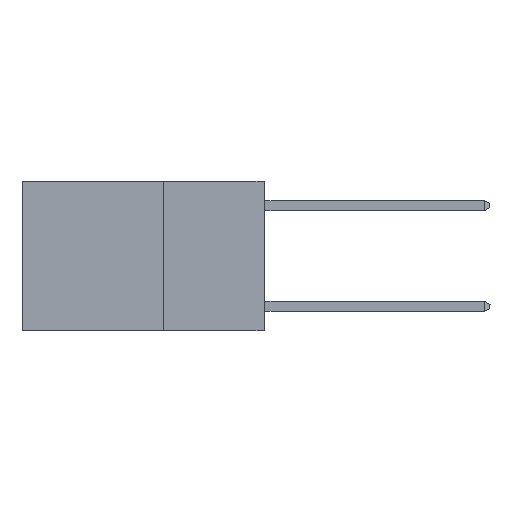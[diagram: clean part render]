
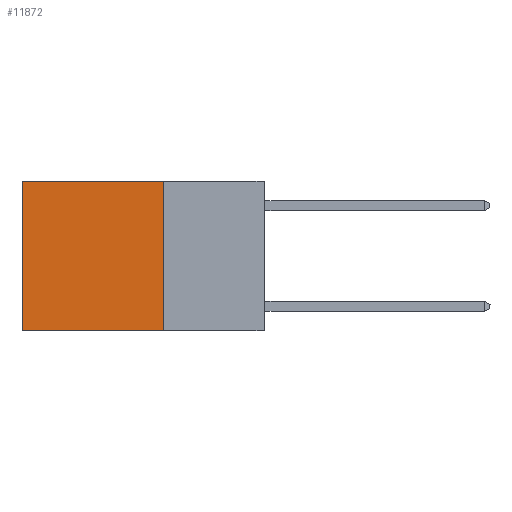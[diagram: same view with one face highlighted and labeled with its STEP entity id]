
A CAD part, left-side view. The second image highlights one B-rep face of the part: STEP entity #11872.
In plain terms, the highlighted planar face has unit normal (-1, 0, 0).
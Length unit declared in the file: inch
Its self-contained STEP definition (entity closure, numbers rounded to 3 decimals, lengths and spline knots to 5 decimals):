
#581 = LINE ( 'NONE', #2000, #25462 ) ;
#1449 = PLANE ( 'NONE',  #12450 ) ;
#1751 = DIRECTION ( 'NONE',  ( 0., 1., 0. ) ) ;
#1859 = LINE ( 'NONE', #28001, #8351 ) ;
#2000 = CARTESIAN_POINT ( 'NONE',  ( 0.2625, 0.6, 0. ) ) ;
#2267 = LINE ( 'NONE', #19824, #20061 ) ;
#4244 = EDGE_CURVE ( 'NONE', #11460, #20288, #2267, .T. ) ;
#4685 = VERTEX_POINT ( 'NONE', #14009 ) ;
#4867 = ORIENTED_EDGE ( 'NONE', *, *, #16510, .T. ) ;
#6562 = CARTESIAN_POINT ( 'NONE',  ( 0.2625, 0.25, 0. ) ) ;
#6848 = VECTOR ( 'NONE', #1751, 39.37008 ) ;
#7389 = FACE_OUTER_BOUND ( 'NONE', #16696, .T. ) ;
#8351 = VECTOR ( 'NONE', #20882, 39.37008 ) ;
#8789 = CARTESIAN_POINT ( 'NONE',  ( 0.2625, 0.25, 0. ) ) ;
#9320 = DIRECTION ( 'NONE',  ( 0., 0., -1. ) ) ;
#10225 = DIRECTION ( 'NONE',  ( 0., 1., 0. ) ) ;
#11220 = DIRECTION ( 'NONE',  ( 1., 0., 0. ) ) ;
#11307 = CARTESIAN_POINT ( 'NONE',  ( 0.2625, 0.6, -0.37 ) ) ;
#11460 = VERTEX_POINT ( 'NONE', #19365 ) ;
#11872 = ADVANCED_FACE ( 'NONE', ( #7389 ), #1449, .F. ) ;
#12450 = AXIS2_PLACEMENT_3D ( 'NONE', #8789, #11220, #27911 ) ;
#12528 = ORIENTED_EDGE ( 'NONE', *, *, #4244, .F. ) ;
#13255 = LINE ( 'NONE', #6562, #6848 ) ;
#14009 = CARTESIAN_POINT ( 'NONE',  ( 0.2625, 0.25, 0. ) ) ;
#14390 = EDGE_CURVE ( 'NONE', #4685, #11460, #1859, .T. ) ;
#14433 = EDGE_CURVE ( 'NONE', #4685, #24748, #13255, .T. ) ;
#16510 = EDGE_CURVE ( 'NONE', #24748, #20288, #581, .T. ) ;
#16696 = EDGE_LOOP ( 'NONE', ( #4867, #12528, #22081, #19444 ) ) ;
#19365 = CARTESIAN_POINT ( 'NONE',  ( 0.2625, 0.25, -0.37 ) ) ;
#19444 = ORIENTED_EDGE ( 'NONE', *, *, #14433, .T. ) ;
#19824 = CARTESIAN_POINT ( 'NONE',  ( 0.2625, 0.25, -0.37 ) ) ;
#20061 = VECTOR ( 'NONE', #10225, 39.37008 ) ;
#20288 = VERTEX_POINT ( 'NONE', #11307 ) ;
#20882 = DIRECTION ( 'NONE',  ( 0., 0., -1. ) ) ;
#22081 = ORIENTED_EDGE ( 'NONE', *, *, #14390, .F. ) ;
#24748 = VERTEX_POINT ( 'NONE', #26087 ) ;
#25462 = VECTOR ( 'NONE', #9320, 39.37008 ) ;
#26087 = CARTESIAN_POINT ( 'NONE',  ( 0.2625, 0.6, 0. ) ) ;
#27911 = DIRECTION ( 'NONE',  ( 0., 0., -1. ) ) ;
#28001 = CARTESIAN_POINT ( 'NONE',  ( 0.2625, 0.25, 0. ) ) ;
